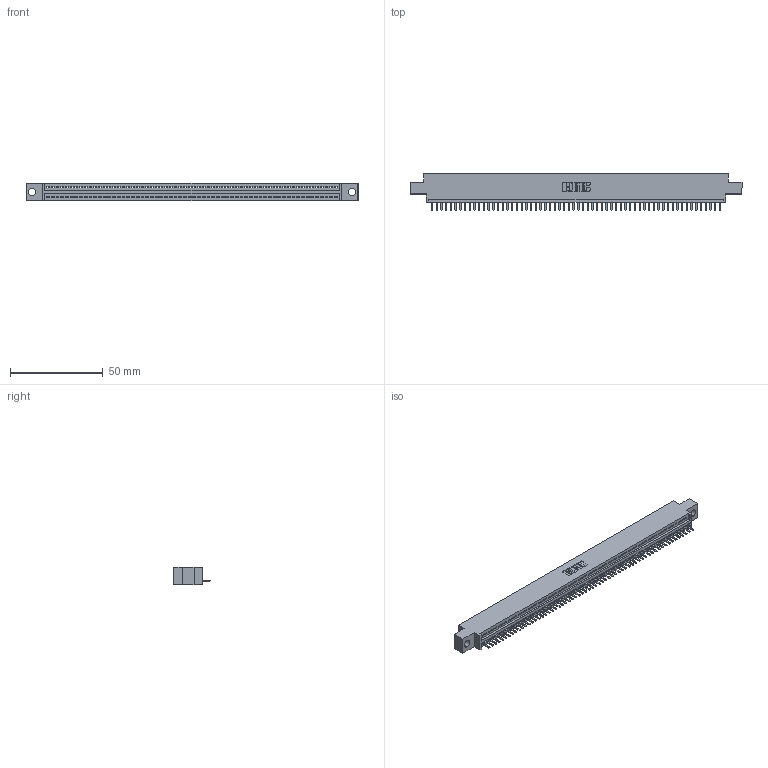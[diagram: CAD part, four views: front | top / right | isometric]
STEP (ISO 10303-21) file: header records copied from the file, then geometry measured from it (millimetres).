
FILE_DESCRIPTION (( 'STEP AP203' ), '1' );
FILE_NAME ('395-062-520-604.STEP', '2019-10-24T16:55:11', ( '' ), ( '' ), 'SwSTEP 2.0', 'SolidWorks 2016', '' );
FILE_SCHEMA (( 'CONFIG_CONTROL_DESIGN' ));
Length unit declared in the file: inch
Products named in the file (3): 345 Part_0.170 Offset - 0.156 Dia-TH; 345-292-001_345-293-120; 395-062-520-604
Assembly tree (63 placements, depth 2):
  395-062-520-604
    345 Part_0.170 Offset - 0.156 Dia-TH
    345-292-001_345-293-120  x62
Bounding box: 178.69 x 19.68 x 9.4 mm (x, y, z)
Volume: 16756.3 mm3; surface area: 21891.3 mm2
Topology: 63 solids, 63 shells, 3974 faces, 11761 edges, 7674 vertices
Faces by surface type: plane 2688, cylinder 1286
Entity records: 44219 total; most frequent: CARTESIAN_POINT 7678, ORIENTED_EDGE 7662, DIRECTION 6663, EDGE_CURVE 3831, VECTOR 3447, LINE 3447, VERTEX_POINT 2550, AXIS2_PLACEMENT_3D 1608
